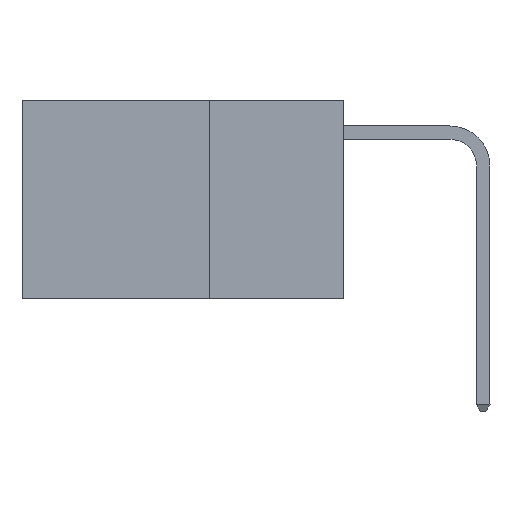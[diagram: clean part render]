
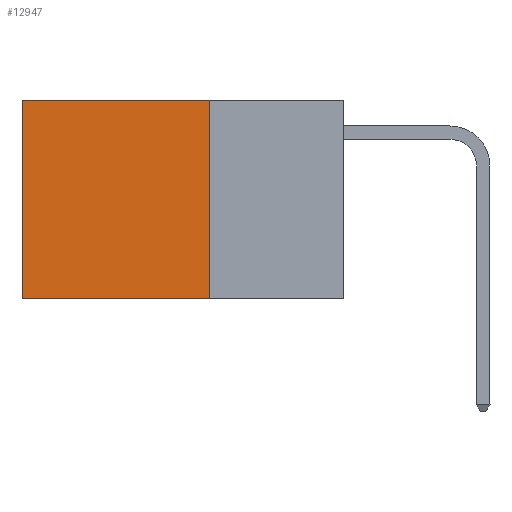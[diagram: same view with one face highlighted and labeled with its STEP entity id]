
A CAD part, left-side view. The second image highlights one B-rep face of the part: STEP entity #12947.
In plain terms, the highlighted planar face has unit normal (-1, 0, 0).
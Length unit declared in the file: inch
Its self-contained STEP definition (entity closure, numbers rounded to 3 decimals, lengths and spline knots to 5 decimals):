
#363 = PLANE ( 'NONE',  #3977 ) ;
#365 = DIRECTION ( 'NONE',  ( 0., 1., 0. ) ) ;
#1132 = ORIENTED_EDGE ( 'NONE', *, *, #4976, .T. ) ;
#1966 = ORIENTED_EDGE ( 'NONE', *, *, #6746, .F. ) ;
#2028 = EDGE_CURVE ( 'NONE', #3975, #7937, #9652, .T. ) ;
#2774 = LINE ( 'NONE', #4634, #10712 ) ;
#2970 = CARTESIAN_POINT ( 'NONE',  ( 0.2625, 0.25, -0.37 ) ) ;
#3642 = CARTESIAN_POINT ( 'NONE',  ( 0.2625, 0.6, -0.37 ) ) ;
#3847 = EDGE_LOOP ( 'NONE', ( #5786, #6290, #1966, #1132 ) ) ;
#3975 = VERTEX_POINT ( 'NONE', #2970 ) ;
#3977 = AXIS2_PLACEMENT_3D ( 'NONE', #11784, #5726, #12769 ) ;
#4634 = CARTESIAN_POINT ( 'NONE',  ( 0.2625, 0.6, 0. ) ) ;
#4712 = VERTEX_POINT ( 'NONE', #10588 ) ;
#4976 = EDGE_CURVE ( 'NONE', #4712, #12613, #8074, .T. ) ;
#5329 = VECTOR ( 'NONE', #7623, 39.37008 ) ;
#5703 = DIRECTION ( 'NONE',  ( 0., 0., -1. ) ) ;
#5726 = DIRECTION ( 'NONE',  ( 1., 0., 0. ) ) ;
#5786 = ORIENTED_EDGE ( 'NONE', *, *, #7893, .T. ) ;
#6290 = ORIENTED_EDGE ( 'NONE', *, *, #2028, .F. ) ;
#6746 = EDGE_CURVE ( 'NONE', #4712, #3975, #11060, .T. ) ;
#7623 = DIRECTION ( 'NONE',  ( 0., 0., -1. ) ) ;
#7893 = EDGE_CURVE ( 'NONE', #12613, #7937, #2774, .T. ) ;
#7937 = VERTEX_POINT ( 'NONE', #3642 ) ;
#8074 = LINE ( 'NONE', #12944, #13106 ) ;
#9652 = LINE ( 'NONE', #12431, #12045 ) ;
#10588 = CARTESIAN_POINT ( 'NONE',  ( 0.2625, 0.25, 0. ) ) ;
#10699 = CARTESIAN_POINT ( 'NONE',  ( 0.2625, 0.6, 0. ) ) ;
#10712 = VECTOR ( 'NONE', #5703, 39.37008 ) ;
#11060 = LINE ( 'NONE', #11657, #5329 ) ;
#11657 = CARTESIAN_POINT ( 'NONE',  ( 0.2625, 0.25, 0. ) ) ;
#11784 = CARTESIAN_POINT ( 'NONE',  ( 0.2625, 0.25, 0. ) ) ;
#11972 = DIRECTION ( 'NONE',  ( 0., 1., 0. ) ) ;
#12045 = VECTOR ( 'NONE', #365, 39.37008 ) ;
#12431 = CARTESIAN_POINT ( 'NONE',  ( 0.2625, 0.25, -0.37 ) ) ;
#12613 = VERTEX_POINT ( 'NONE', #10699 ) ;
#12769 = DIRECTION ( 'NONE',  ( 0., 0., -1. ) ) ;
#12927 = FACE_OUTER_BOUND ( 'NONE', #3847, .T. ) ;
#12944 = CARTESIAN_POINT ( 'NONE',  ( 0.2625, 0.25, 0. ) ) ;
#12947 = ADVANCED_FACE ( 'NONE', ( #12927 ), #363, .F. ) ;
#13106 = VECTOR ( 'NONE', #11972, 39.37008 ) ;
